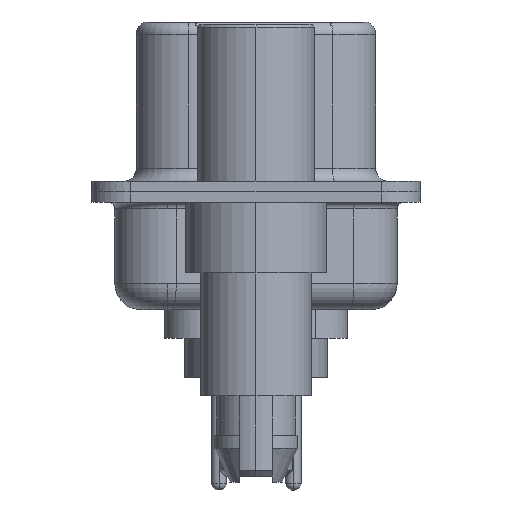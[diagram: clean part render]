
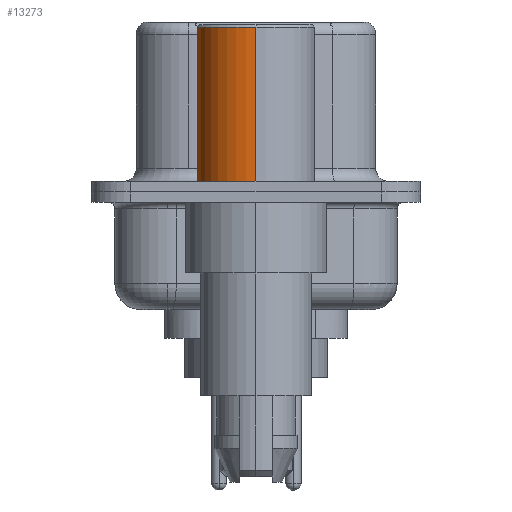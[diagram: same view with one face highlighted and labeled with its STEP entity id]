
A CAD part, left-side view. The second image highlights one B-rep face of the part: STEP entity #13273.
In plain terms, the highlighted cylindrical face has radius 2.25 mm (diameter 4.5 mm), a partial arc.
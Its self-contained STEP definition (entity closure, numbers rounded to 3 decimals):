
#633 = CARTESIAN_POINT ( 'NONE',  ( -2.25, 0., 0.581 ) ) ;
#937 = EDGE_CURVE ( 'NONE', #10963, #21319, #13166, .T. ) ;
#1028 = CARTESIAN_POINT ( 'NONE',  ( -2.25, 0., 6.3 ) ) ;
#2109 = VECTOR ( 'NONE', #11121, 1000. ) ;
#2625 = DIRECTION ( 'NONE',  ( 0., 0., 1. ) ) ;
#2767 = CIRCLE ( 'NONE', #20838, 2.25 ) ;
#4132 = CARTESIAN_POINT ( 'NONE',  ( 2.25, 0., 0.581 ) ) ;
#5311 = CYLINDRICAL_SURFACE ( 'NONE', #7430, 2.25 ) ;
#6827 = EDGE_LOOP ( 'NONE', ( #13514, #10521, #11805, #14993 ) ) ;
#7423 = VERTEX_POINT ( 'NONE', #14554 ) ;
#7430 = AXIS2_PLACEMENT_3D ( 'NONE', #11423, #14947, #7918 ) ;
#7918 = DIRECTION ( 'NONE',  ( 1., 0., 0. ) ) ;
#9550 = DIRECTION ( 'NONE',  ( 0., 0., 1. ) ) ;
#9794 = DIRECTION ( 'NONE',  ( 0., 0., 1. ) ) ;
#10139 = EDGE_CURVE ( 'NONE', #7423, #21319, #21246, .T. ) ;
#10521 = ORIENTED_EDGE ( 'NONE', *, *, #937, .T. ) ;
#10963 = VERTEX_POINT ( 'NONE', #17234 ) ;
#11121 = DIRECTION ( 'NONE',  ( 0., 0., 1. ) ) ;
#11423 = CARTESIAN_POINT ( 'NONE',  ( 0., 0., 0.581 ) ) ;
#11805 = ORIENTED_EDGE ( 'NONE', *, *, #10139, .F. ) ;
#13144 = CARTESIAN_POINT ( 'NONE',  ( 0., 0., 6.3 ) ) ;
#13166 = LINE ( 'NONE', #633, #21928 ) ;
#13273 = ADVANCED_FACE ( 'NONE', ( #19301 ), #5311, .T. ) ;
#13514 = ORIENTED_EDGE ( 'NONE', *, *, #15439, .T. ) ;
#14554 = CARTESIAN_POINT ( 'NONE',  ( 2.25, 0., 6.3 ) ) ;
#14888 = DIRECTION ( 'NONE',  ( 1., 0., 0. ) ) ;
#14947 = DIRECTION ( 'NONE',  ( 0., 0., 1. ) ) ;
#14993 = ORIENTED_EDGE ( 'NONE', *, *, #21967, .F. ) ;
#15439 = EDGE_CURVE ( 'NONE', #22221, #10963, #2767, .T. ) ;
#17234 = CARTESIAN_POINT ( 'NONE',  ( -2.25, 0., 0.4 ) ) ;
#18508 = AXIS2_PLACEMENT_3D ( 'NONE', #13144, #2625, #14888 ) ;
#19301 = FACE_OUTER_BOUND ( 'NONE', #6827, .T. ) ;
#20071 = CARTESIAN_POINT ( 'NONE',  ( 0., 0., 0.4 ) ) ;
#20728 = LINE ( 'NONE', #4132, #2109 ) ;
#20838 = AXIS2_PLACEMENT_3D ( 'NONE', #20071, #9550, #21849 ) ;
#21246 = CIRCLE ( 'NONE', #18508, 2.25 ) ;
#21319 = VERTEX_POINT ( 'NONE', #1028 ) ;
#21849 = DIRECTION ( 'NONE',  ( 1., 0., 0. ) ) ;
#21928 = VECTOR ( 'NONE', #9794, 1000. ) ;
#21967 = EDGE_CURVE ( 'NONE', #22221, #7423, #20728, .T. ) ;
#22221 = VERTEX_POINT ( 'NONE', #22341 ) ;
#22341 = CARTESIAN_POINT ( 'NONE',  ( 2.25, 0., 0.4 ) ) ;
